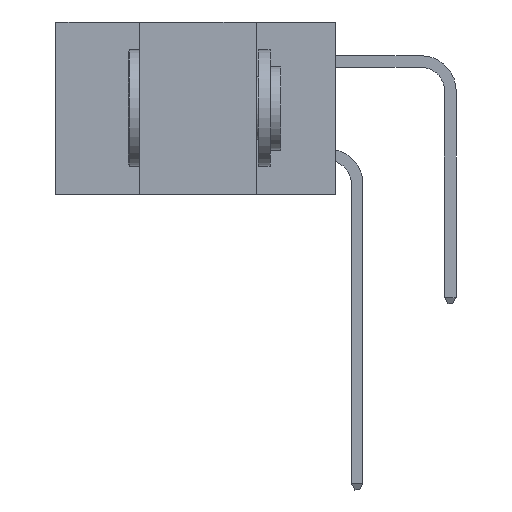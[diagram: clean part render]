
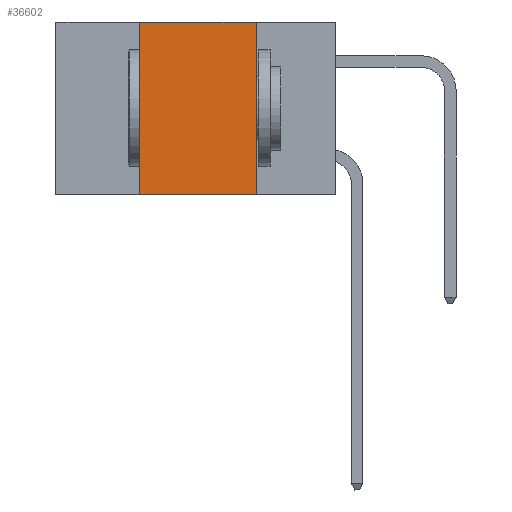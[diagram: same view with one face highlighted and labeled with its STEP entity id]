
A CAD part, left-side view. The second image highlights one B-rep face of the part: STEP entity #36602.
In plain terms, the highlighted planar face has unit normal (-1, 0, 0).
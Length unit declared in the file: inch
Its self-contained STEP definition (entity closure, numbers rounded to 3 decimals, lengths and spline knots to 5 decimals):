
#506 = VECTOR ( 'NONE', #32751, 39.37008 ) ;
#841 = ORIENTED_EDGE ( 'NONE', *, *, #27285, .F. ) ;
#1330 = CARTESIAN_POINT ( 'NONE',  ( 0., 0.17, -0.37 ) ) ;
#2782 = LINE ( 'NONE', #39226, #35681 ) ;
#5143 = VERTEX_POINT ( 'NONE', #39652 ) ;
#8139 = DIRECTION ( 'NONE',  ( 1., 0., 0. ) ) ;
#8239 = LINE ( 'NONE', #16144, #35156 ) ;
#9191 = EDGE_CURVE ( 'NONE', #5143, #36604, #25162, .T. ) ;
#9811 = DIRECTION ( 'NONE',  ( 0., -1., 0. ) ) ;
#11466 = CARTESIAN_POINT ( 'NONE',  ( 0., 0.6, 0. ) ) ;
#12294 = AXIS2_PLACEMENT_3D ( 'NONE', #11466, #8139, #18065 ) ;
#13752 = PLANE ( 'NONE',  #12294 ) ;
#14695 = VECTOR ( 'NONE', #21214, 39.37008 ) ;
#15838 = VERTEX_POINT ( 'NONE', #24463 ) ;
#16144 = CARTESIAN_POINT ( 'NONE',  ( 0., 0.6, -0.37 ) ) ;
#16535 = VERTEX_POINT ( 'NONE', #21632 ) ;
#17363 = ORIENTED_EDGE ( 'NONE', *, *, #9191, .F. ) ;
#18065 = DIRECTION ( 'NONE',  ( 0., 0., -1. ) ) ;
#19953 = ORIENTED_EDGE ( 'NONE', *, *, #30669, .F. ) ;
#21214 = DIRECTION ( 'NONE',  ( 0., 0., -1. ) ) ;
#21471 = FACE_OUTER_BOUND ( 'NONE', #28492, .T. ) ;
#21632 = CARTESIAN_POINT ( 'NONE',  ( 0., 0.42, -0.37 ) ) ;
#22957 = LINE ( 'NONE', #23565, #506 ) ;
#23565 = CARTESIAN_POINT ( 'NONE',  ( 0., 0.42, 0. ) ) ;
#24463 = CARTESIAN_POINT ( 'NONE',  ( 0., 0.42, 0. ) ) ;
#25162 = LINE ( 'NONE', #30664, #14695 ) ;
#26449 = DIRECTION ( 'NONE',  ( 0., -1., 0. ) ) ;
#26820 = ORIENTED_EDGE ( 'NONE', *, *, #30464, .T. ) ;
#27285 = EDGE_CURVE ( 'NONE', #16535, #15838, #22957, .T. ) ;
#28492 = EDGE_LOOP ( 'NONE', ( #17363, #19953, #841, #26820 ) ) ;
#30464 = EDGE_CURVE ( 'NONE', #16535, #36604, #8239, .T. ) ;
#30664 = CARTESIAN_POINT ( 'NONE',  ( 0., 0.17, 0. ) ) ;
#30669 = EDGE_CURVE ( 'NONE', #15838, #5143, #2782, .T. ) ;
#32751 = DIRECTION ( 'NONE',  ( 0., 0., 1. ) ) ;
#35156 = VECTOR ( 'NONE', #9811, 39.37008 ) ;
#35681 = VECTOR ( 'NONE', #26449, 39.37008 ) ;
#36602 = ADVANCED_FACE ( 'NONE', ( #21471 ), #13752, .F. ) ;
#36604 = VERTEX_POINT ( 'NONE', #1330 ) ;
#39226 = CARTESIAN_POINT ( 'NONE',  ( 0., 0.6, 0. ) ) ;
#39652 = CARTESIAN_POINT ( 'NONE',  ( 0., 0.17, 0. ) ) ;
